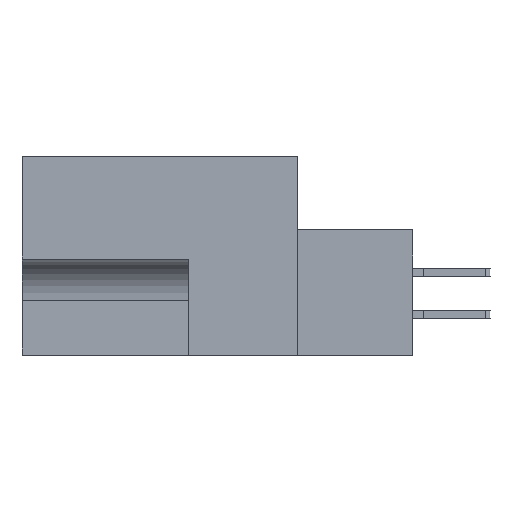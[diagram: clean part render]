
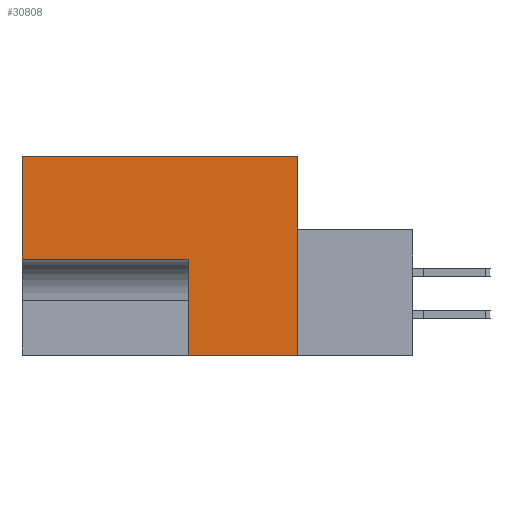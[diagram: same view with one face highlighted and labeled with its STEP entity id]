
A CAD part, left-side view. The second image highlights one B-rep face of the part: STEP entity #30808.
In plain terms, the highlighted planar face has unit normal (-1, 0, 0).
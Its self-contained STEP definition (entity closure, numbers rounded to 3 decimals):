
#928 = LINE ( 'NONE', #37984, #15932 ) ;
#2336 = DIRECTION ( 'NONE',  ( 0., 1., 0. ) ) ;
#2678 = LINE ( 'NONE', #5851, #15827 ) ;
#5640 = CARTESIAN_POINT ( 'NONE',  ( 0., 11.506, 0. ) ) ;
#5851 = CARTESIAN_POINT ( 'NONE',  ( 0., 20.955, -15.088 ) ) ;
#6748 = CARTESIAN_POINT ( 'NONE',  ( 0., 0., -15.088 ) ) ;
#8617 = VECTOR ( 'NONE', #11142, 1000. ) ;
#9125 = VERTEX_POINT ( 'NONE', #31487 ) ;
#10990 = ORIENTED_EDGE ( 'NONE', *, *, #37678, .F. ) ;
#11142 = DIRECTION ( 'NONE',  ( 0., 1., 0. ) ) ;
#11770 = CARTESIAN_POINT ( 'NONE',  ( 0., 0., 0. ) ) ;
#12391 = LINE ( 'NONE', #50994, #8617 ) ;
#13376 = EDGE_CURVE ( 'NONE', #9125, #28055, #13777, .T. ) ;
#13777 = LINE ( 'NONE', #5640, #19370 ) ;
#14292 = CARTESIAN_POINT ( 'NONE',  ( 0., 0., 0. ) ) ;
#15164 = CARTESIAN_POINT ( 'NONE',  ( 0., 0., 0. ) ) ;
#15460 = DIRECTION ( 'NONE',  ( 1., 0., 0. ) ) ;
#15685 = LINE ( 'NONE', #15164, #40700 ) ;
#15827 = VECTOR ( 'NONE', #41850, 1000. ) ;
#15838 = DIRECTION ( 'NONE',  ( 0., 0., -1. ) ) ;
#15932 = VECTOR ( 'NONE', #29767, 1000. ) ;
#16592 = CARTESIAN_POINT ( 'NONE',  ( 0., 8.255, -15.088 ) ) ;
#16981 = VERTEX_POINT ( 'NONE', #6748 ) ;
#17348 = EDGE_CURVE ( 'NONE', #51645, #21699, #928, .T. ) ;
#18331 = VECTOR ( 'NONE', #2336, 1000. ) ;
#18937 = EDGE_LOOP ( 'NONE', ( #32156, #50873, #44559, #10990, #23062, #25360 ) ) ;
#19370 = VECTOR ( 'NONE', #40777, 1000. ) ;
#21699 = VERTEX_POINT ( 'NONE', #35152 ) ;
#22200 = EDGE_CURVE ( 'NONE', #16981, #51645, #12391, .T. ) ;
#23062 = ORIENTED_EDGE ( 'NONE', *, *, #37758, .F. ) ;
#25360 = ORIENTED_EDGE ( 'NONE', *, *, #17348, .F. ) ;
#27475 = PLANE ( 'NONE',  #38313 ) ;
#28055 = VERTEX_POINT ( 'NONE', #14292 ) ;
#29767 = DIRECTION ( 'NONE',  ( 0., 0., 1. ) ) ;
#30217 = VERTEX_POINT ( 'NONE', #47377 ) ;
#30808 = ADVANCED_FACE ( 'NONE', ( #42757 ), #27475, .F. ) ;
#31487 = CARTESIAN_POINT ( 'NONE',  ( 0., 20.955, 0. ) ) ;
#32156 = ORIENTED_EDGE ( 'NONE', *, *, #22200, .F. ) ;
#35152 = CARTESIAN_POINT ( 'NONE',  ( 0., 8.255, -7.772 ) ) ;
#37678 = EDGE_CURVE ( 'NONE', #30217, #9125, #2678, .T. ) ;
#37758 = EDGE_CURVE ( 'NONE', #21699, #30217, #45869, .T. ) ;
#37984 = CARTESIAN_POINT ( 'NONE',  ( 0., 8.255, -15.088 ) ) ;
#38313 = AXIS2_PLACEMENT_3D ( 'NONE', #11770, #15460, #47237 ) ;
#39157 = EDGE_CURVE ( 'NONE', #28055, #16981, #15685, .T. ) ;
#40700 = VECTOR ( 'NONE', #15838, 1000. ) ;
#40777 = DIRECTION ( 'NONE',  ( 0., -1., 0. ) ) ;
#41850 = DIRECTION ( 'NONE',  ( 0., 0., 1. ) ) ;
#42757 = FACE_OUTER_BOUND ( 'NONE', #18937, .T. ) ;
#44559 = ORIENTED_EDGE ( 'NONE', *, *, #13376, .F. ) ;
#45869 = LINE ( 'NONE', #50212, #18331 ) ;
#47237 = DIRECTION ( 'NONE',  ( 0., 0., -1. ) ) ;
#47377 = CARTESIAN_POINT ( 'NONE',  ( 0., 20.955, -7.772 ) ) ;
#50212 = CARTESIAN_POINT ( 'NONE',  ( 0., 8.255, -7.772 ) ) ;
#50873 = ORIENTED_EDGE ( 'NONE', *, *, #39157, .F. ) ;
#50994 = CARTESIAN_POINT ( 'NONE',  ( 0., -8.814, -15.088 ) ) ;
#51645 = VERTEX_POINT ( 'NONE', #16592 ) ;
